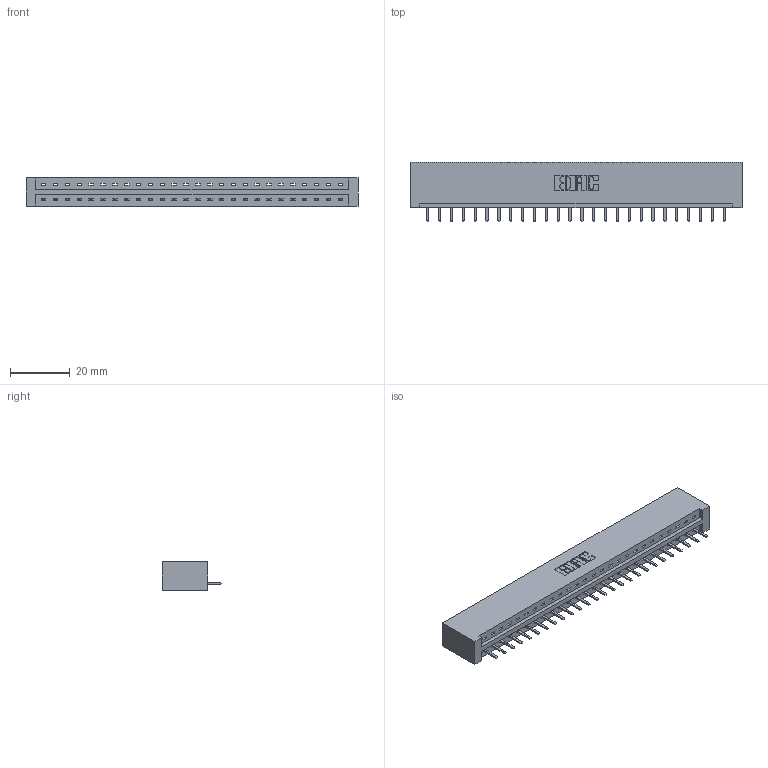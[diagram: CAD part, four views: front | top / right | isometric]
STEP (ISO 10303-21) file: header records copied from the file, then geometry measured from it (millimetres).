
FILE_DESCRIPTION (( 'STEP AP203' ), '1' );
FILE_NAME ('387-026-520-101.STEP', '2018-09-15T21:21:19', ( '' ), ( '' ), 'SwSTEP 2.0', 'SolidWorks 2016', '' );
FILE_SCHEMA (( 'CONFIG_CONTROL_DESIGN' ));
Length unit declared in the file: inch
Products named in the file (3): 345-292-001_345-293-120; 387-026-520-101; 337 Part_No Mounting Lugs
Assembly tree (27 placements, depth 2):
  387-026-520-101
    337 Part_No Mounting Lugs
    345-292-001_345-293-120  x26
Bounding box: 110.9 x 20.02 x 9.4 mm (x, y, z)
Volume: 11989.5 mm3; surface area: 12012.8 mm2
Topology: 27 solids, 27 shells, 1822 faces, 5383 edges, 3518 vertices
Faces by surface type: plane 1314, cylinder 508
Entity records: 21233 total; most frequent: CARTESIAN_POINT 3716, ORIENTED_EDGE 3666, DIRECTION 3141, EDGE_CURVE 1833, VECTOR 1709, LINE 1709, VERTEX_POINT 1218, AXIS2_PLACEMENT_3D 716
